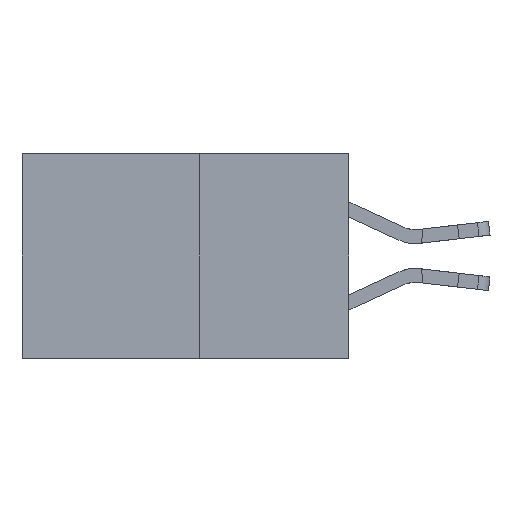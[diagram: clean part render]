
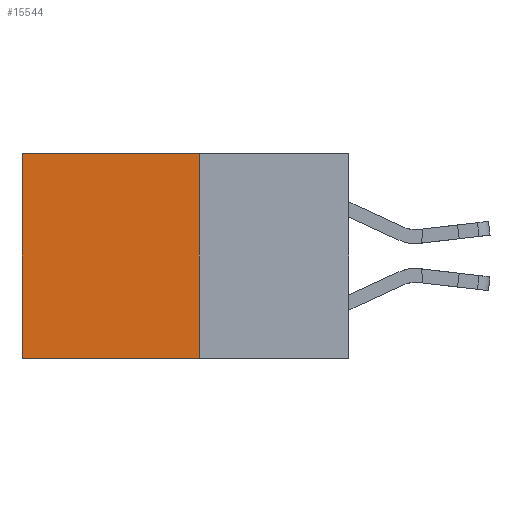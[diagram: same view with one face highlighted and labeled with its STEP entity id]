
A CAD part, left-side view. The second image highlights one B-rep face of the part: STEP entity #15544.
In plain terms, the highlighted planar face has unit normal (-1, 0, 0).
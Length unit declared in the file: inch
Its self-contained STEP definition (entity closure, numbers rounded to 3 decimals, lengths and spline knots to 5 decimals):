
#46 = LINE ( 'NONE', #525, #5698 ) ;
#525 = CARTESIAN_POINT ( 'NONE',  ( 0.277, 0.27, 0. ) ) ;
#667 = CARTESIAN_POINT ( 'NONE',  ( 0.277, 0.27, -0.37 ) ) ;
#716 = CARTESIAN_POINT ( 'NONE',  ( 0.277, 0.27, -0.37 ) ) ;
#783 = DIRECTION ( 'NONE',  ( 0., 1., 0. ) ) ;
#1565 = CARTESIAN_POINT ( 'NONE',  ( 0.277, 0.27, -0.37 ) ) ;
#1716 = LINE ( 'NONE', #716, #7796 ) ;
#2136 = DIRECTION ( 'NONE',  ( 1., 0., 0. ) ) ;
#3472 = EDGE_LOOP ( 'NONE', ( #3596, #5500, #11434, #13282 ) ) ;
#3596 = ORIENTED_EDGE ( 'NONE', *, *, #5239, .T. ) ;
#4604 = VERTEX_POINT ( 'NONE', #1565 ) ;
#5239 = EDGE_CURVE ( 'NONE', #13298, #5383, #8806, .T. ) ;
#5383 = VERTEX_POINT ( 'NONE', #13367 ) ;
#5500 = ORIENTED_EDGE ( 'NONE', *, *, #6525, .F. ) ;
#5698 = VECTOR ( 'NONE', #12625, 39.37008 ) ;
#5716 = CARTESIAN_POINT ( 'NONE',  ( 0.277, 0.27, -0.37 ) ) ;
#6305 = VECTOR ( 'NONE', #14651, 39.37008 ) ;
#6487 = VECTOR ( 'NONE', #10392, 39.37008 ) ;
#6525 = EDGE_CURVE ( 'NONE', #4604, #5383, #1716, .T. ) ;
#6857 = LINE ( 'NONE', #667, #6487 ) ;
#7796 = VECTOR ( 'NONE', #783, 39.37008 ) ;
#8806 = LINE ( 'NONE', #14596, #6305 ) ;
#9047 = EDGE_CURVE ( 'NONE', #15480, #4604, #6857, .T. ) ;
#9274 = AXIS2_PLACEMENT_3D ( 'NONE', #5716, #2136, #10649 ) ;
#9453 = PLANE ( 'NONE',  #9274 ) ;
#10392 = DIRECTION ( 'NONE',  ( 0., 0., -1. ) ) ;
#10649 = DIRECTION ( 'NONE',  ( 0., 0., -1. ) ) ;
#11434 = ORIENTED_EDGE ( 'NONE', *, *, #9047, .F. ) ;
#11596 = FACE_OUTER_BOUND ( 'NONE', #3472, .T. ) ;
#12625 = DIRECTION ( 'NONE',  ( 0., 1., 0. ) ) ;
#12865 = CARTESIAN_POINT ( 'NONE',  ( 0.277, 0.27, 0. ) ) ;
#13282 = ORIENTED_EDGE ( 'NONE', *, *, #15293, .T. ) ;
#13298 = VERTEX_POINT ( 'NONE', #15046 ) ;
#13367 = CARTESIAN_POINT ( 'NONE',  ( 0.277, 0.59, -0.37 ) ) ;
#14596 = CARTESIAN_POINT ( 'NONE',  ( 0.277, 0.59, -0.37 ) ) ;
#14651 = DIRECTION ( 'NONE',  ( 0., 0., -1. ) ) ;
#15046 = CARTESIAN_POINT ( 'NONE',  ( 0.277, 0.59, 0. ) ) ;
#15293 = EDGE_CURVE ( 'NONE', #15480, #13298, #46, .T. ) ;
#15480 = VERTEX_POINT ( 'NONE', #12865 ) ;
#15544 = ADVANCED_FACE ( 'NONE', ( #11596 ), #9453, .F. ) ;
